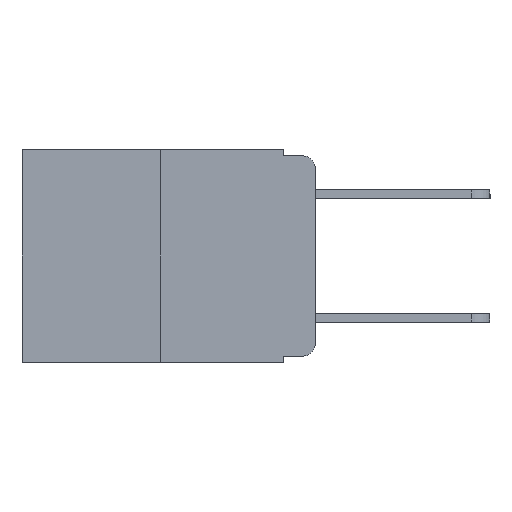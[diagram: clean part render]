
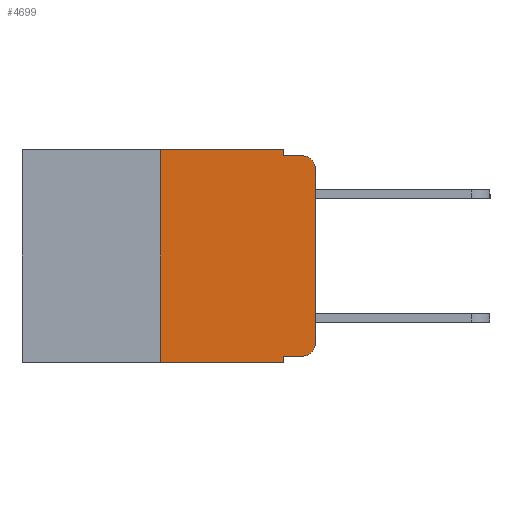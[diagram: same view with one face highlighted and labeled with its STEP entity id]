
A CAD part, left-side view. The second image highlights one B-rep face of the part: STEP entity #4699.
In plain terms, the highlighted planar face has unit normal (-1, 0, 0).
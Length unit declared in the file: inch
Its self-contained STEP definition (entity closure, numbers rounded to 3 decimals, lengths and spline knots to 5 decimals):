
#113 = ORIENTED_EDGE ( 'NONE', *, *, #8327, .F. ) ;
#150 = DIRECTION ( 'NONE',  ( 0., 0., 1. ) ) ;
#224 = CARTESIAN_POINT ( 'NONE',  ( 0., 0.051, 0. ) ) ;
#234 = VERTEX_POINT ( 'NONE', #6651 ) ;
#647 = LINE ( 'NONE', #15271, #10692 ) ;
#791 = ORIENTED_EDGE ( 'NONE', *, *, #8895, .T. ) ;
#1060 = CARTESIAN_POINT ( 'NONE',  ( 0., 0.25, -0.343 ) ) ;
#1507 = DIRECTION ( 'NONE',  ( 0., -1., 0. ) ) ;
#1540 = ORIENTED_EDGE ( 'NONE', *, *, #8896, .F. ) ;
#1610 = VERTEX_POINT ( 'NONE', #13414 ) ;
#1635 = CARTESIAN_POINT ( 'NONE',  ( 0., 0.25, 0. ) ) ;
#1699 = CARTESIAN_POINT ( 'NONE',  ( 0., 0.02, -0.03 ) ) ;
#1740 = CARTESIAN_POINT ( 'NONE',  ( 0., 0., -0.313 ) ) ;
#1925 = ORIENTED_EDGE ( 'NONE', *, *, #8924, .F. ) ;
#2324 = CARTESIAN_POINT ( 'NONE',  ( 0., 0.02, -0.333 ) ) ;
#2549 = VERTEX_POINT ( 'NONE', #2324 ) ;
#2901 = ORIENTED_EDGE ( 'NONE', *, *, #8951, .T. ) ;
#3104 = DIRECTION ( 'NONE',  ( 0., 0., -1. ) ) ;
#3158 = DIRECTION ( 'NONE',  ( 0., 0., -1. ) ) ;
#3538 = LINE ( 'NONE', #13248, #9916 ) ;
#3774 = VECTOR ( 'NONE', #1507, 39.37008 ) ;
#3966 = VECTOR ( 'NONE', #4458, 39.37008 ) ;
#4021 = AXIS2_PLACEMENT_3D ( 'NONE', #1699, #10703, #3104 ) ;
#4164 = VERTEX_POINT ( 'NONE', #1740 ) ;
#4212 = CARTESIAN_POINT ( 'NONE',  ( 0., 0., -0.03 ) ) ;
#4338 = VERTEX_POINT ( 'NONE', #7572 ) ;
#4405 = CIRCLE ( 'NONE', #4021, 0.02 ) ;
#4458 = DIRECTION ( 'NONE',  ( 0., 0., -1. ) ) ;
#4529 = ORIENTED_EDGE ( 'NONE', *, *, #8873, .T. ) ;
#4699 = ADVANCED_FACE ( 'NONE', ( #6049 ), #7482, .F. ) ;
#4824 = LINE ( 'NONE', #224, #16035 ) ;
#4936 = AXIS2_PLACEMENT_3D ( 'NONE', #14300, #7076, #15420 ) ;
#5103 = ORIENTED_EDGE ( 'NONE', *, *, #8921, .F. ) ;
#5587 = ORIENTED_EDGE ( 'NONE', *, *, #8373, .T. ) ;
#5634 = VERTEX_POINT ( 'NONE', #8589 ) ;
#6049 = FACE_OUTER_BOUND ( 'NONE', #12364, .T. ) ;
#6463 = ORIENTED_EDGE ( 'NONE', *, *, #8899, .F. ) ;
#6651 = CARTESIAN_POINT ( 'NONE',  ( 0., 0.051, -0.01 ) ) ;
#6789 = VERTEX_POINT ( 'NONE', #1635 ) ;
#7076 = DIRECTION ( 'NONE',  ( -1., 0., 0. ) ) ;
#7135 = VERTEX_POINT ( 'NONE', #4212 ) ;
#7307 = VECTOR ( 'NONE', #150, 39.37008 ) ;
#7349 = VERTEX_POINT ( 'NONE', #1060 ) ;
#7482 = PLANE ( 'NONE',  #15804 ) ;
#7572 = CARTESIAN_POINT ( 'NONE',  ( 0., 0.051, -0.333 ) ) ;
#8216 = CARTESIAN_POINT ( 'NONE',  ( 0., 0.25, 0. ) ) ;
#8327 = EDGE_CURVE ( 'NONE', #6789, #1610, #8331, .T. ) ;
#8331 = LINE ( 'NONE', #11708, #14328 ) ;
#8373 = EDGE_CURVE ( 'NONE', #7349, #5634, #10902, .T. ) ;
#8589 = CARTESIAN_POINT ( 'NONE',  ( 0., 0.051, -0.343 ) ) ;
#8873 = EDGE_CURVE ( 'NONE', #4164, #7135, #14151, .T. ) ;
#8890 = CARTESIAN_POINT ( 'NONE',  ( 0., 0.473, 0. ) ) ;
#8895 = EDGE_CURVE ( 'NONE', #7135, #11747, #4405, .T. ) ;
#8896 = EDGE_CURVE ( 'NONE', #234, #11747, #647, .T. ) ;
#8899 = EDGE_CURVE ( 'NONE', #1610, #234, #13840, .T. ) ;
#8921 = EDGE_CURVE ( 'NONE', #7349, #6789, #10320, .T. ) ;
#8924 = EDGE_CURVE ( 'NONE', #4338, #5634, #4824, .T. ) ;
#8927 = DIRECTION ( 'NONE',  ( 0., 0., -1. ) ) ;
#8931 = EDGE_CURVE ( 'NONE', #4338, #2549, #3538, .T. ) ;
#8951 = EDGE_CURVE ( 'NONE', #2549, #4164, #12820, .T. ) ;
#9055 = ORIENTED_EDGE ( 'NONE', *, *, #8931, .T. ) ;
#9390 = CARTESIAN_POINT ( 'NONE',  ( 0., 0., 0. ) ) ;
#9456 = CARTESIAN_POINT ( 'NONE',  ( 0., 0.051, 0. ) ) ;
#9916 = VECTOR ( 'NONE', #14262, 39.37008 ) ;
#10320 = LINE ( 'NONE', #8216, #7307 ) ;
#10692 = VECTOR ( 'NONE', #13145, 39.37008 ) ;
#10703 = DIRECTION ( 'NONE',  ( -1., 0., 0. ) ) ;
#10902 = LINE ( 'NONE', #14037, #3774 ) ;
#11074 = VECTOR ( 'NONE', #14169, 39.37008 ) ;
#11708 = CARTESIAN_POINT ( 'NONE',  ( 0., 0.473, 0. ) ) ;
#11747 = VERTEX_POINT ( 'NONE', #14917 ) ;
#12364 = EDGE_LOOP ( 'NONE', ( #4529, #791, #1540, #6463, #113, #5103, #5587, #1925, #9055, #2901 ) ) ;
#12820 = CIRCLE ( 'NONE', #4936, 0.02 ) ;
#12947 = DIRECTION ( 'NONE',  ( 0., -1., 0. ) ) ;
#13145 = DIRECTION ( 'NONE',  ( 0., -1., 0. ) ) ;
#13248 = CARTESIAN_POINT ( 'NONE',  ( 0., 0.051, -0.333 ) ) ;
#13414 = CARTESIAN_POINT ( 'NONE',  ( 0., 0.051, 0. ) ) ;
#13840 = LINE ( 'NONE', #9456, #3966 ) ;
#14037 = CARTESIAN_POINT ( 'NONE',  ( 0., 0.473, -0.343 ) ) ;
#14151 = LINE ( 'NONE', #9390, #11074 ) ;
#14169 = DIRECTION ( 'NONE',  ( 0., 0., 1. ) ) ;
#14262 = DIRECTION ( 'NONE',  ( 0., -1., 0. ) ) ;
#14300 = CARTESIAN_POINT ( 'NONE',  ( 0., 0.02, -0.313 ) ) ;
#14328 = VECTOR ( 'NONE', #12947, 39.37008 ) ;
#14784 = DIRECTION ( 'NONE',  ( 1., 0., 0. ) ) ;
#14917 = CARTESIAN_POINT ( 'NONE',  ( 0., 0.02, -0.01 ) ) ;
#15271 = CARTESIAN_POINT ( 'NONE',  ( 0., 0.051, -0.01 ) ) ;
#15420 = DIRECTION ( 'NONE',  ( 0., 0., -1. ) ) ;
#15804 = AXIS2_PLACEMENT_3D ( 'NONE', #8890, #14784, #8927 ) ;
#16035 = VECTOR ( 'NONE', #3158, 39.37008 ) ;
